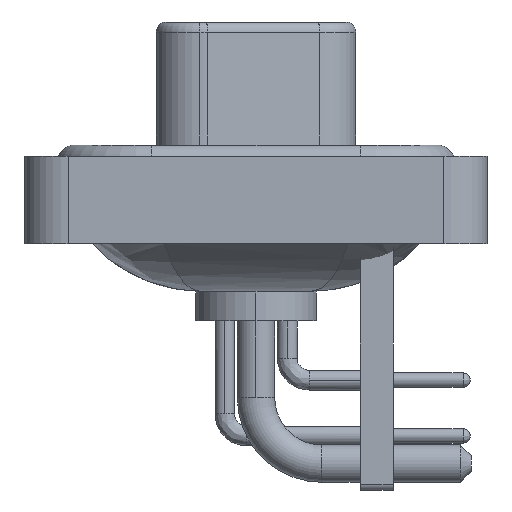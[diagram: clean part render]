
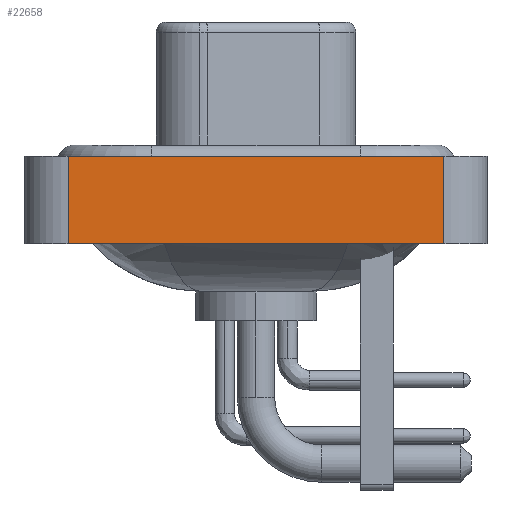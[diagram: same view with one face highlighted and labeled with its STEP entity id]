
A CAD part, left-side view. The second image highlights one B-rep face of the part: STEP entity #22658.
In plain terms, the highlighted planar face has unit normal (-1, 0, 0).
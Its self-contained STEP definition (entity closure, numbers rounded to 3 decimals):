
#1190 = DIRECTION ( 'NONE',  ( 0., 0., 1. ) ) ;
#1492 = ORIENTED_EDGE ( 'NONE', *, *, #6753, .T. ) ;
#2661 = LINE ( 'NONE', #13558, #12000 ) ;
#2995 = EDGE_LOOP ( 'NONE', ( #23558, #6446, #20056, #1492 ) ) ;
#3604 = EDGE_CURVE ( 'NONE', #13677, #26383, #11950, .T. ) ;
#5247 = VECTOR ( 'NONE', #1190, 1000. ) ;
#5459 = VERTEX_POINT ( 'NONE', #5554 ) ;
#5554 = CARTESIAN_POINT ( 'NONE',  ( -7.35, -8.55, -3.6 ) ) ;
#6446 = ORIENTED_EDGE ( 'NONE', *, *, #12992, .F. ) ;
#6470 = CARTESIAN_POINT ( 'NONE',  ( -7.35, -8.55, -3.6 ) ) ;
#6753 = EDGE_CURVE ( 'NONE', #13677, #5459, #2661, .T. ) ;
#9448 = DIRECTION ( 'NONE',  ( 0., -1., 0. ) ) ;
#10240 = AXIS2_PLACEMENT_3D ( 'NONE', #6470, #15398, #15112 ) ;
#11674 = CARTESIAN_POINT ( 'NONE',  ( -7.35, 8.55, -3.6 ) ) ;
#11950 = LINE ( 'NONE', #15942, #5247 ) ;
#12000 = VECTOR ( 'NONE', #9448, 1000. ) ;
#12294 = VERTEX_POINT ( 'NONE', #25392 ) ;
#12992 = EDGE_CURVE ( 'NONE', #26383, #12294, #26475, .T. ) ;
#13516 = EDGE_CURVE ( 'NONE', #5459, #12294, #19791, .T. ) ;
#13556 = PLANE ( 'NONE',  #10240 ) ;
#13558 = CARTESIAN_POINT ( 'NONE',  ( -7.35, -8.55, -3.6 ) ) ;
#13573 = CARTESIAN_POINT ( 'NONE',  ( -7.35, -8.55, 0.4 ) ) ;
#13677 = VERTEX_POINT ( 'NONE', #11674 ) ;
#15112 = DIRECTION ( 'NONE',  ( 0., 0., 1. ) ) ;
#15398 = DIRECTION ( 'NONE',  ( -1., 0., 0. ) ) ;
#15802 = DIRECTION ( 'NONE',  ( 0., 0., 1. ) ) ;
#15942 = CARTESIAN_POINT ( 'NONE',  ( -7.35, 8.55, -3.6 ) ) ;
#17551 = DIRECTION ( 'NONE',  ( 0., -1., 0. ) ) ;
#19062 = VECTOR ( 'NONE', #17551, 1000. ) ;
#19791 = LINE ( 'NONE', #21925, #20445 ) ;
#20056 = ORIENTED_EDGE ( 'NONE', *, *, #3604, .F. ) ;
#20445 = VECTOR ( 'NONE', #15802, 1000. ) ;
#21925 = CARTESIAN_POINT ( 'NONE',  ( -7.35, -8.55, -3.6 ) ) ;
#22157 = CARTESIAN_POINT ( 'NONE',  ( -7.35, 8.55, 0.4 ) ) ;
#22658 = ADVANCED_FACE ( 'NONE', ( #26034 ), #13556, .T. ) ;
#23558 = ORIENTED_EDGE ( 'NONE', *, *, #13516, .T. ) ;
#25392 = CARTESIAN_POINT ( 'NONE',  ( -7.35, -8.55, 0.4 ) ) ;
#26034 = FACE_OUTER_BOUND ( 'NONE', #2995, .T. ) ;
#26383 = VERTEX_POINT ( 'NONE', #22157 ) ;
#26475 = LINE ( 'NONE', #13573, #19062 ) ;
